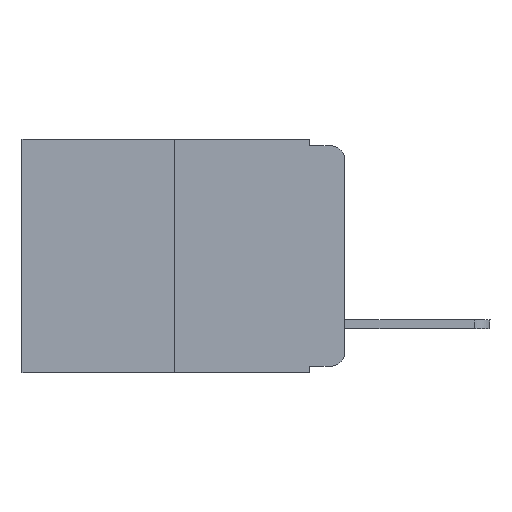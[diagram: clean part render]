
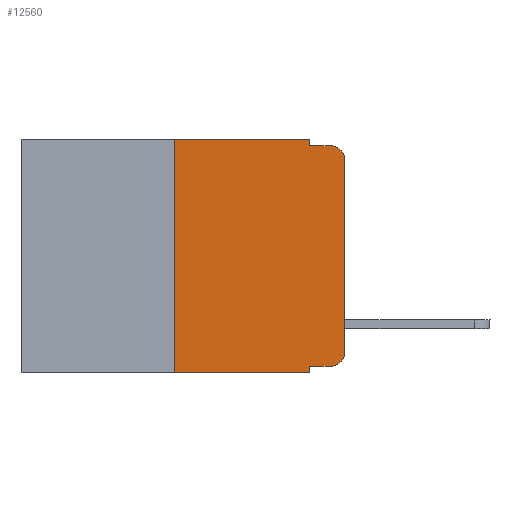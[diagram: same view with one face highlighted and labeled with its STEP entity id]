
A CAD part, left-side view. The second image highlights one B-rep face of the part: STEP entity #12560.
In plain terms, the highlighted planar face has unit normal (-1, 0, 0).
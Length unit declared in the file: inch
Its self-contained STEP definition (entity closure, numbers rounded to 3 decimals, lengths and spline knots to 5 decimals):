
#459 = CARTESIAN_POINT ( 'NONE',  ( 0., 0., -0.313 ) ) ;
#831 = CARTESIAN_POINT ( 'NONE',  ( 0., 0.25, 0. ) ) ;
#1045 = VECTOR ( 'NONE', #9802, 39.37008 ) ;
#1173 = ORIENTED_EDGE ( 'NONE', *, *, #10821, .F. ) ;
#1229 = VERTEX_POINT ( 'NONE', #9774 ) ;
#1244 = DIRECTION ( 'NONE',  ( 0., 0., -1. ) ) ;
#1338 = LINE ( 'NONE', #6859, #1045 ) ;
#1381 = CARTESIAN_POINT ( 'NONE',  ( 0., 0.051, 0. ) ) ;
#1799 = CARTESIAN_POINT ( 'NONE',  ( 0., 0.051, -0.343 ) ) ;
#1983 = CARTESIAN_POINT ( 'NONE',  ( 0., 0., -0.03 ) ) ;
#2052 = VECTOR ( 'NONE', #11745, 39.37008 ) ;
#2135 = FACE_OUTER_BOUND ( 'NONE', #14740, .T. ) ;
#2155 = LINE ( 'NONE', #831, #13324 ) ;
#2338 = AXIS2_PLACEMENT_3D ( 'NONE', #8792, #7373, #10045 ) ;
#2449 = VECTOR ( 'NONE', #2870, 39.37008 ) ;
#2870 = DIRECTION ( 'NONE',  ( 0., -1., 0. ) ) ;
#2885 = LINE ( 'NONE', #1381, #10387 ) ;
#3059 = DIRECTION ( 'NONE',  ( 0., 0., -1. ) ) ;
#3516 = DIRECTION ( 'NONE',  ( 0., 0., -1. ) ) ;
#3596 = CARTESIAN_POINT ( 'NONE',  ( 0., 0.02, -0.313 ) ) ;
#3686 = LINE ( 'NONE', #5744, #5591 ) ;
#3731 = DIRECTION ( 'NONE',  ( 1., 0., 0. ) ) ;
#3997 = ORIENTED_EDGE ( 'NONE', *, *, #6297, .T. ) ;
#4744 = LINE ( 'NONE', #5892, #8658 ) ;
#5012 = EDGE_CURVE ( 'NONE', #10677, #5145, #1338, .T. ) ;
#5145 = VERTEX_POINT ( 'NONE', #12655 ) ;
#5166 = LINE ( 'NONE', #17120, #2052 ) ;
#5202 = CIRCLE ( 'NONE', #2338, 0.02 ) ;
#5274 = CARTESIAN_POINT ( 'NONE',  ( 0., 0.25, -0.343 ) ) ;
#5591 = VECTOR ( 'NONE', #3059, 39.37008 ) ;
#5744 = CARTESIAN_POINT ( 'NONE',  ( 0., 0.051, 0. ) ) ;
#5750 = DIRECTION ( 'NONE',  ( 0., 0., -1. ) ) ;
#5892 = CARTESIAN_POINT ( 'NONE',  ( 0., 0., 0. ) ) ;
#6234 = CARTESIAN_POINT ( 'NONE',  ( 0., 0.473, 0. ) ) ;
#6285 = DIRECTION ( 'NONE',  ( 0., -1., 0. ) ) ;
#6297 = EDGE_CURVE ( 'NONE', #7622, #13882, #4744, .T. ) ;
#6319 = ORIENTED_EDGE ( 'NONE', *, *, #16244, .T. ) ;
#6799 = LINE ( 'NONE', #15008, #2449 ) ;
#6859 = CARTESIAN_POINT ( 'NONE',  ( 0., 0.473, 0. ) ) ;
#6969 = EDGE_CURVE ( 'NONE', #5145, #1229, #2885, .T. ) ;
#7236 = CARTESIAN_POINT ( 'NONE',  ( 0., 0.051, -0.333 ) ) ;
#7373 = DIRECTION ( 'NONE',  ( -1., 0., 0. ) ) ;
#7476 = CARTESIAN_POINT ( 'NONE',  ( 0., 0.02, -0.333 ) ) ;
#7567 = PLANE ( 'NONE',  #11026 ) ;
#7622 = VERTEX_POINT ( 'NONE', #459 ) ;
#7635 = LINE ( 'NONE', #13077, #16915 ) ;
#7676 = DIRECTION ( 'NONE',  ( 0., 0., 1. ) ) ;
#8500 = ORIENTED_EDGE ( 'NONE', *, *, #6969, .F. ) ;
#8658 = VECTOR ( 'NONE', #10169, 39.37008 ) ;
#8705 = EDGE_CURVE ( 'NONE', #1229, #17208, #6799, .T. ) ;
#8792 = CARTESIAN_POINT ( 'NONE',  ( 0., 0.02, -0.03 ) ) ;
#9774 = CARTESIAN_POINT ( 'NONE',  ( 0., 0.051, -0.01 ) ) ;
#9802 = DIRECTION ( 'NONE',  ( 0., -1., 0. ) ) ;
#10045 = DIRECTION ( 'NONE',  ( 0., 0., -1. ) ) ;
#10169 = DIRECTION ( 'NONE',  ( 0., 0., 1. ) ) ;
#10305 = ORIENTED_EDGE ( 'NONE', *, *, #14750, .T. ) ;
#10387 = VECTOR ( 'NONE', #5750, 39.37008 ) ;
#10677 = VERTEX_POINT ( 'NONE', #15195 ) ;
#10809 = ORIENTED_EDGE ( 'NONE', *, *, #17502, .F. ) ;
#10821 = EDGE_CURVE ( 'NONE', #15380, #10677, #2155, .T. ) ;
#11026 = AXIS2_PLACEMENT_3D ( 'NONE', #6234, #3731, #1244 ) ;
#11745 = DIRECTION ( 'NONE',  ( 0., -1., 0. ) ) ;
#12360 = CIRCLE ( 'NONE', #16354, 0.02 ) ;
#12560 = ADVANCED_FACE ( 'NONE', ( #2135 ), #7567, .F. ) ;
#12655 = CARTESIAN_POINT ( 'NONE',  ( 0., 0.051, 0. ) ) ;
#12699 = ORIENTED_EDGE ( 'NONE', *, *, #14500, .T. ) ;
#12747 = ORIENTED_EDGE ( 'NONE', *, *, #8705, .F. ) ;
#13077 = CARTESIAN_POINT ( 'NONE',  ( 0., 0.473, -0.343 ) ) ;
#13293 = CARTESIAN_POINT ( 'NONE',  ( 0., 0.02, -0.01 ) ) ;
#13324 = VECTOR ( 'NONE', #7676, 39.37008 ) ;
#13870 = VERTEX_POINT ( 'NONE', #7236 ) ;
#13882 = VERTEX_POINT ( 'NONE', #1983 ) ;
#14375 = VERTEX_POINT ( 'NONE', #7476 ) ;
#14500 = EDGE_CURVE ( 'NONE', #13870, #14375, #5166, .T. ) ;
#14740 = EDGE_LOOP ( 'NONE', ( #3997, #10305, #12747, #8500, #17615, #1173, #6319, #10809, #12699, #15447 ) ) ;
#14750 = EDGE_CURVE ( 'NONE', #13882, #17208, #5202, .T. ) ;
#15008 = CARTESIAN_POINT ( 'NONE',  ( 0., 0.051, -0.01 ) ) ;
#15195 = CARTESIAN_POINT ( 'NONE',  ( 0., 0.25, 0. ) ) ;
#15380 = VERTEX_POINT ( 'NONE', #5274 ) ;
#15447 = ORIENTED_EDGE ( 'NONE', *, *, #16596, .T. ) ;
#16244 = EDGE_CURVE ( 'NONE', #15380, #16901, #7635, .T. ) ;
#16354 = AXIS2_PLACEMENT_3D ( 'NONE', #3596, #17250, #3516 ) ;
#16596 = EDGE_CURVE ( 'NONE', #14375, #7622, #12360, .T. ) ;
#16901 = VERTEX_POINT ( 'NONE', #1799 ) ;
#16915 = VECTOR ( 'NONE', #6285, 39.37008 ) ;
#17120 = CARTESIAN_POINT ( 'NONE',  ( 0., 0.051, -0.333 ) ) ;
#17208 = VERTEX_POINT ( 'NONE', #13293 ) ;
#17250 = DIRECTION ( 'NONE',  ( -1., 0., 0. ) ) ;
#17502 = EDGE_CURVE ( 'NONE', #13870, #16901, #3686, .T. ) ;
#17615 = ORIENTED_EDGE ( 'NONE', *, *, #5012, .F. ) ;
